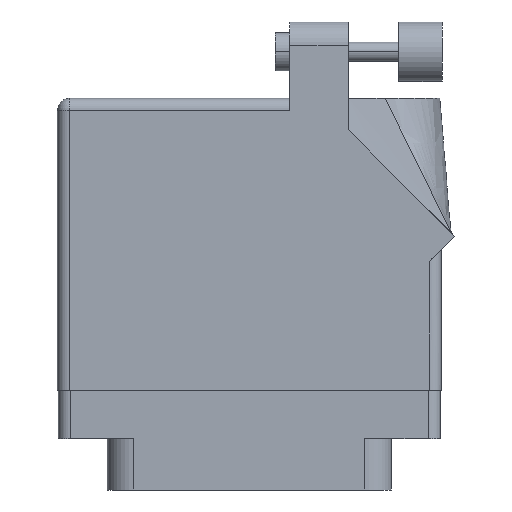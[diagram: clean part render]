
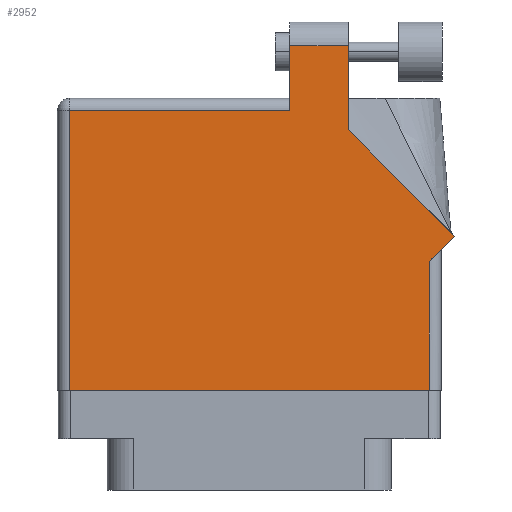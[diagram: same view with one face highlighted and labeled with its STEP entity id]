
A CAD part, front view. The second image highlights one B-rep face of the part: STEP entity #2952.
In plain terms, the highlighted face is planar.
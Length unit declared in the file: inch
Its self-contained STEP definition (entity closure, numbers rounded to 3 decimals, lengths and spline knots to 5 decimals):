
#503 = CARTESIAN_POINT ( 'NONE',  ( 0.519, 1.705, 0.455 ) ) ;
#1510 = VECTOR ( 'NONE', #25614, 39.37008 ) ;
#1962 = ORIENTED_EDGE ( 'NONE', *, *, #27162, .T. ) ;
#2233 = DIRECTION ( 'NONE',  ( 1., 0., 0. ) ) ;
#2952 = ADVANCED_FACE ( 'NONE', ( #28641 ), #16897, .F. ) ;
#3129 = CARTESIAN_POINT ( 'NONE',  ( 0.212, 1.705, 0.455 ) ) ;
#3586 = VERTEX_POINT ( 'NONE', #27359 ) ;
#3947 = VERTEX_POINT ( 'NONE', #503 ) ;
#4346 = ORIENTED_EDGE ( 'NONE', *, *, #9720, .T. ) ;
#4472 = CARTESIAN_POINT ( 'NONE',  ( 0.212, 1.705, 0.455 ) ) ;
#4547 = DIRECTION ( 'NONE',  ( 0., 1., 0. ) ) ;
#4588 = ORIENTED_EDGE ( 'NONE', *, *, #4822, .T. ) ;
#4633 = VECTOR ( 'NONE', #4547, 39.37008 ) ;
#4822 = EDGE_CURVE ( 'NONE', #13268, #15151, #20010, .T. ) ;
#6558 = VECTOR ( 'NONE', #2233, 39.37008 ) ;
#6710 = LINE ( 'NONE', #13279, #13615 ) ;
#6857 = VECTOR ( 'NONE', #26439, 39.37008 ) ;
#8275 = CARTESIAN_POINT ( 'NONE',  ( 0.943, 0.575, 0.455 ) ) ;
#8874 = EDGE_CURVE ( 'NONE', #3947, #30281, #29342, .T. ) ;
#8966 = EDGE_LOOP ( 'NONE', ( #19425, #15322, #25235, #33162, #1962, #4588, #32495, #21380, #4346 ) ) ;
#9720 = EDGE_CURVE ( 'NONE', #26017, #15891, #33210, .T. ) ;
#9768 = EDGE_CURVE ( 'NONE', #30281, #11820, #24492, .T. ) ;
#11386 = DIRECTION ( 'NONE',  ( -0.707, 0.707, 0. ) ) ;
#11820 = VERTEX_POINT ( 'NONE', #35839 ) ;
#12948 = EDGE_CURVE ( 'NONE', #23074, #26017, #14486, .T. ) ;
#13268 = VERTEX_POINT ( 'NONE', #25826 ) ;
#13279 = CARTESIAN_POINT ( 'NONE',  ( 0.943, 0.637, 0.455 ) ) ;
#13615 = VECTOR ( 'NONE', #16206, 39.37008 ) ;
#13967 = DIRECTION ( 'NONE',  ( -1., 0., 0. ) ) ;
#14486 = LINE ( 'NONE', #15267, #22267 ) ;
#15151 = VERTEX_POINT ( 'NONE', #19812 ) ;
#15267 = CARTESIAN_POINT ( 'NONE',  ( 1.005, 0.637, 0.455 ) ) ;
#15322 = ORIENTED_EDGE ( 'NONE', *, *, #8874, .T. ) ;
#15752 = CARTESIAN_POINT ( 'NONE',  ( 1.07571, 0.70771, 0.455 ) ) ;
#15891 = VERTEX_POINT ( 'NONE', #17159 ) ;
#16206 = DIRECTION ( 'NONE',  ( 0., 1., 0. ) ) ;
#16897 = PLANE ( 'NONE',  #34419 ) ;
#17131 = DIRECTION ( 'NONE',  ( 0., 0., -1. ) ) ;
#17159 = CARTESIAN_POINT ( 'NONE',  ( 0.519, 1.26442, 0.455 ) ) ;
#17779 = EDGE_CURVE ( 'NONE', #15891, #3947, #19379, .T. ) ;
#17856 = DIRECTION ( 'NONE',  ( 0., -1., 0. ) ) ;
#17929 = CARTESIAN_POINT ( 'NONE',  ( -0.943, -0.1, 0.455 ) ) ;
#18391 = VECTOR ( 'NONE', #17856, 39.37008 ) ;
#18634 = CARTESIAN_POINT ( 'NONE',  ( -1.005, -0.1, 0.455 ) ) ;
#19379 = LINE ( 'NONE', #35405, #4633 ) ;
#19425 = ORIENTED_EDGE ( 'NONE', *, *, #17779, .T. ) ;
#19812 = CARTESIAN_POINT ( 'NONE',  ( 0.943, -0.1, 0.455 ) ) ;
#20010 = LINE ( 'NONE', #18634, #6558 ) ;
#20622 = DIRECTION ( 'NONE',  ( 0.707, 0.707, 0. ) ) ;
#21380 = ORIENTED_EDGE ( 'NONE', *, *, #12948, .T. ) ;
#22267 = VECTOR ( 'NONE', #20622, 39.37008 ) ;
#22375 = DIRECTION ( 'NONE',  ( -1., 0., 0. ) ) ;
#23074 = VERTEX_POINT ( 'NONE', #8275 ) ;
#24492 = LINE ( 'NONE', #34189, #18391 ) ;
#25235 = ORIENTED_EDGE ( 'NONE', *, *, #9768, .T. ) ;
#25614 = DIRECTION ( 'NONE',  ( -1., 0., 0. ) ) ;
#25673 = CARTESIAN_POINT ( 'NONE',  ( -1.005, 1.368, 0.455 ) ) ;
#25799 = VECTOR ( 'NONE', #11386, 39.37008 ) ;
#25826 = CARTESIAN_POINT ( 'NONE',  ( -0.943, -0.1, 0.455 ) ) ;
#26017 = VERTEX_POINT ( 'NONE', #15752 ) ;
#26439 = DIRECTION ( 'NONE',  ( 0., -1., 0. ) ) ;
#27162 = EDGE_CURVE ( 'NONE', #3586, #13268, #29935, .T. ) ;
#27359 = CARTESIAN_POINT ( 'NONE',  ( -0.943, 1.368, 0.455 ) ) ;
#28102 = CARTESIAN_POINT ( 'NONE',  ( 1.07571, 0.70771, 0.455 ) ) ;
#28641 = FACE_OUTER_BOUND ( 'NONE', #8966, .T. ) ;
#29149 = EDGE_CURVE ( 'NONE', #15151, #23074, #6710, .T. ) ;
#29323 = EDGE_CURVE ( 'NONE', #11820, #3586, #31052, .T. ) ;
#29342 = LINE ( 'NONE', #3129, #1510 ) ;
#29935 = LINE ( 'NONE', #17929, #6857 ) ;
#30281 = VERTEX_POINT ( 'NONE', #4472 ) ;
#31052 = LINE ( 'NONE', #25673, #31508 ) ;
#31156 = CARTESIAN_POINT ( 'NONE',  ( -1.005, 1.43, 0.455 ) ) ;
#31508 = VECTOR ( 'NONE', #22375, 39.37008 ) ;
#32495 = ORIENTED_EDGE ( 'NONE', *, *, #29149, .T. ) ;
#33162 = ORIENTED_EDGE ( 'NONE', *, *, #29323, .T. ) ;
#33210 = LINE ( 'NONE', #28102, #25799 ) ;
#34189 = CARTESIAN_POINT ( 'NONE',  ( 0.212, 1.43, 0.455 ) ) ;
#34419 = AXIS2_PLACEMENT_3D ( 'NONE', #31156, #17131, #13967 ) ;
#35405 = CARTESIAN_POINT ( 'NONE',  ( 0.519, 1.26442, 0.455 ) ) ;
#35839 = CARTESIAN_POINT ( 'NONE',  ( 0.212, 1.368, 0.455 ) ) ;
